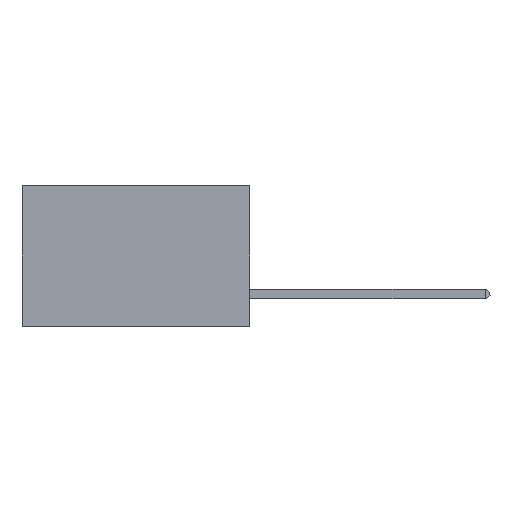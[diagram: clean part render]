
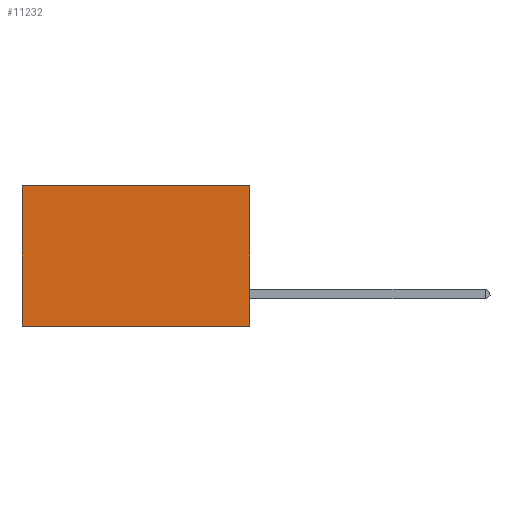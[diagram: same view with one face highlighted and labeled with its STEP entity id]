
A CAD part, left-side view. The second image highlights one B-rep face of the part: STEP entity #11232.
In plain terms, the highlighted planar face has unit normal (-1, 0, 0).
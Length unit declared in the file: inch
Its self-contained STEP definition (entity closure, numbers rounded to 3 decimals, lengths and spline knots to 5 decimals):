
#1248 = EDGE_CURVE ( 'NONE', #9634, #16924, #13053, .T. ) ;
#1521 = DIRECTION ( 'NONE',  ( 0., 1., 0. ) ) ;
#1535 = EDGE_CURVE ( 'NONE', #16924, #16601, #12827, .T. ) ;
#2257 = AXIS2_PLACEMENT_3D ( 'NONE', #13733, #15427, #6560 ) ;
#3383 = CARTESIAN_POINT ( 'NONE',  ( 0.2875, 0., -0.37 ) ) ;
#4438 = CARTESIAN_POINT ( 'NONE',  ( 0.2875, 0., 0. ) ) ;
#4601 = VERTEX_POINT ( 'NONE', #6604 ) ;
#4818 = EDGE_CURVE ( 'NONE', #9634, #4601, #18485, .T. ) ;
#5092 = ORIENTED_EDGE ( 'NONE', *, *, #1535, .T. ) ;
#6086 = ORIENTED_EDGE ( 'NONE', *, *, #10926, .F. ) ;
#6560 = DIRECTION ( 'NONE',  ( 0., 0., -1. ) ) ;
#6604 = CARTESIAN_POINT ( 'NONE',  ( 0.2875, 0., -0.37 ) ) ;
#7440 = CARTESIAN_POINT ( 'NONE',  ( 0.2875, 0., 0. ) ) ;
#7686 = DIRECTION ( 'NONE',  ( 0., 0., -1. ) ) ;
#8246 = DIRECTION ( 'NONE',  ( 0., 0., -1. ) ) ;
#8258 = ORIENTED_EDGE ( 'NONE', *, *, #4818, .F. ) ;
#9602 = LINE ( 'NONE', #3383, #18091 ) ;
#9634 = VERTEX_POINT ( 'NONE', #4438 ) ;
#9965 = CARTESIAN_POINT ( 'NONE',  ( 0.2875, 0.6, 0. ) ) ;
#10926 = EDGE_CURVE ( 'NONE', #4601, #16601, #9602, .T. ) ;
#11232 = ADVANCED_FACE ( 'NONE', ( #17605 ), #12527, .F. ) ;
#11831 = VECTOR ( 'NONE', #8246, 39.37008 ) ;
#12505 = CARTESIAN_POINT ( 'NONE',  ( 0.2875, 0., 0. ) ) ;
#12527 = PLANE ( 'NONE',  #2257 ) ;
#12827 = LINE ( 'NONE', #16420, #18381 ) ;
#13053 = LINE ( 'NONE', #7440, #14172 ) ;
#13604 = DIRECTION ( 'NONE',  ( 0., 1., 0. ) ) ;
#13733 = CARTESIAN_POINT ( 'NONE',  ( 0.2875, 0., 0. ) ) ;
#14172 = VECTOR ( 'NONE', #1521, 39.37008 ) ;
#15427 = DIRECTION ( 'NONE',  ( 1., 0., 0. ) ) ;
#15807 = CARTESIAN_POINT ( 'NONE',  ( 0.2875, 0.6, -0.37 ) ) ;
#16293 = ORIENTED_EDGE ( 'NONE', *, *, #1248, .T. ) ;
#16420 = CARTESIAN_POINT ( 'NONE',  ( 0.2875, 0.6, 0. ) ) ;
#16601 = VERTEX_POINT ( 'NONE', #15807 ) ;
#16924 = VERTEX_POINT ( 'NONE', #9965 ) ;
#17479 = EDGE_LOOP ( 'NONE', ( #5092, #6086, #8258, #16293 ) ) ;
#17605 = FACE_OUTER_BOUND ( 'NONE', #17479, .T. ) ;
#18091 = VECTOR ( 'NONE', #13604, 39.37008 ) ;
#18381 = VECTOR ( 'NONE', #7686, 39.37008 ) ;
#18485 = LINE ( 'NONE', #12505, #11831 ) ;
